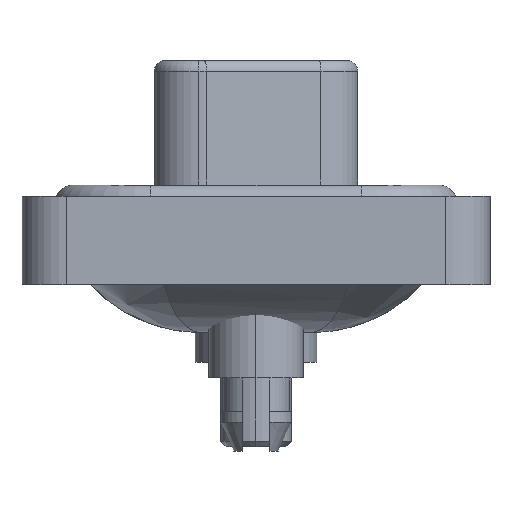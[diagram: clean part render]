
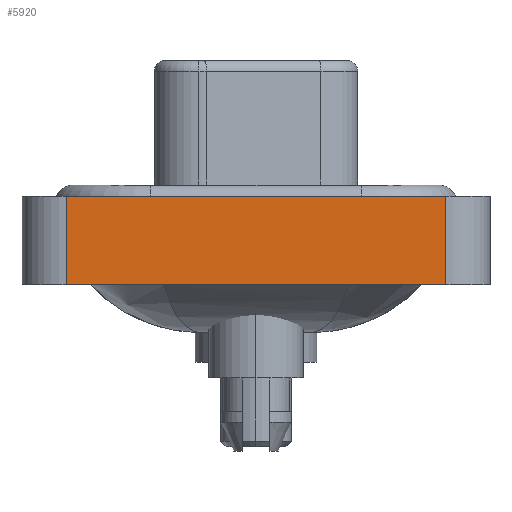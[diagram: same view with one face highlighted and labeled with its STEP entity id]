
A CAD part, left-side view. The second image highlights one B-rep face of the part: STEP entity #5920.
In plain terms, the highlighted planar face has unit normal (-1, 0, 0).
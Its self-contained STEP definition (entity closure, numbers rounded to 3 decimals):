
#96 = VERTEX_POINT ( 'NONE', #3088 ) ;
#743 = DIRECTION ( 'NONE',  ( -1., 0., 0. ) ) ;
#762 = LINE ( 'NONE', #13130, #10126 ) ;
#958 = LINE ( 'NONE', #11811, #7829 ) ;
#1638 = CARTESIAN_POINT ( 'NONE',  ( -7.3, -8.55, -3.6 ) ) ;
#2043 = ORIENTED_EDGE ( 'NONE', *, *, #13013, .F. ) ;
#2278 = DIRECTION ( 'NONE',  ( 0., -1., 0. ) ) ;
#3088 = CARTESIAN_POINT ( 'NONE',  ( -7.3, -8.55, -3.6 ) ) ;
#3273 = LINE ( 'NONE', #8444, #7734 ) ;
#3369 = CARTESIAN_POINT ( 'NONE',  ( -7.3, -8.55, 0.4 ) ) ;
#3428 = EDGE_CURVE ( 'NONE', #96, #8399, #3273, .T. ) ;
#3878 = CARTESIAN_POINT ( 'NONE',  ( -7.3, -8.55, -3.6 ) ) ;
#3967 = DIRECTION ( 'NONE',  ( 0., 0., 1. ) ) ;
#5920 = ADVANCED_FACE ( 'NONE', ( #14626 ), #12914, .T. ) ;
#5976 = EDGE_LOOP ( 'NONE', ( #10022, #2043, #17774, #13577 ) ) ;
#6605 = EDGE_CURVE ( 'NONE', #11533, #16152, #762, .T. ) ;
#7734 = VECTOR ( 'NONE', #3967, 1000. ) ;
#7742 = DIRECTION ( 'NONE',  ( 0., -1., 0. ) ) ;
#7829 = VECTOR ( 'NONE', #2278, 1000. ) ;
#8346 = EDGE_CURVE ( 'NONE', #11533, #96, #15527, .T. ) ;
#8399 = VERTEX_POINT ( 'NONE', #3369 ) ;
#8444 = CARTESIAN_POINT ( 'NONE',  ( -7.3, -8.55, -3.6 ) ) ;
#9818 = VECTOR ( 'NONE', #7742, 1000. ) ;
#10022 = ORIENTED_EDGE ( 'NONE', *, *, #3428, .T. ) ;
#10126 = VECTOR ( 'NONE', #19292, 1000. ) ;
#11418 = CARTESIAN_POINT ( 'NONE',  ( -7.3, 8.55, -3.6 ) ) ;
#11533 = VERTEX_POINT ( 'NONE', #11418 ) ;
#11811 = CARTESIAN_POINT ( 'NONE',  ( -7.3, -8.55, 0.4 ) ) ;
#12914 = PLANE ( 'NONE',  #19777 ) ;
#13013 = EDGE_CURVE ( 'NONE', #16152, #8399, #958, .T. ) ;
#13130 = CARTESIAN_POINT ( 'NONE',  ( -7.3, 8.55, -3.6 ) ) ;
#13577 = ORIENTED_EDGE ( 'NONE', *, *, #8346, .T. ) ;
#14626 = FACE_OUTER_BOUND ( 'NONE', #5976, .T. ) ;
#15527 = LINE ( 'NONE', #1638, #9818 ) ;
#16137 = DIRECTION ( 'NONE',  ( 0., 0., 1. ) ) ;
#16152 = VERTEX_POINT ( 'NONE', #17342 ) ;
#17342 = CARTESIAN_POINT ( 'NONE',  ( -7.3, 8.55, 0.4 ) ) ;
#17774 = ORIENTED_EDGE ( 'NONE', *, *, #6605, .F. ) ;
#19292 = DIRECTION ( 'NONE',  ( 0., 0., 1. ) ) ;
#19777 = AXIS2_PLACEMENT_3D ( 'NONE', #3878, #743, #16137 ) ;
